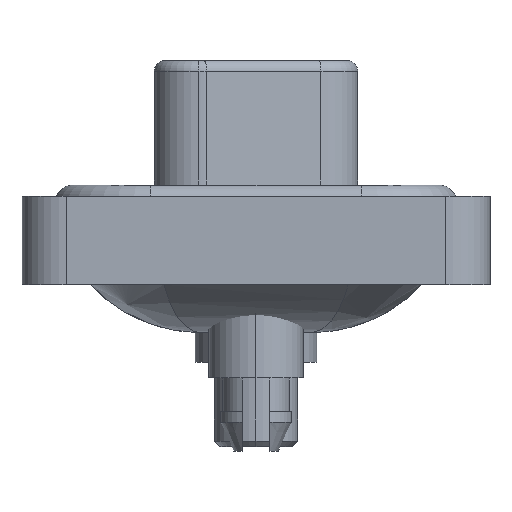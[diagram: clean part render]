
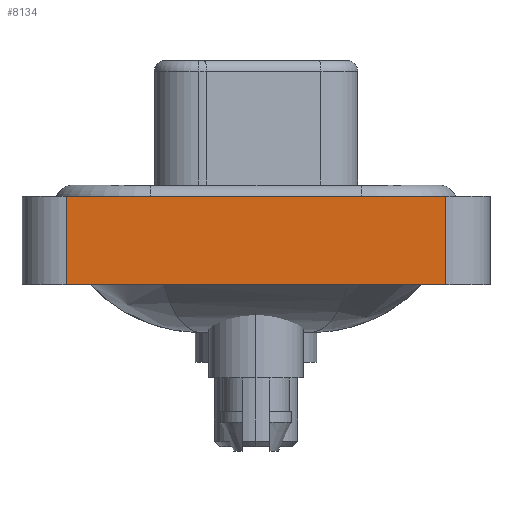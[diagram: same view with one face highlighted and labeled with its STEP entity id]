
A CAD part, left-side view. The second image highlights one B-rep face of the part: STEP entity #8134.
In plain terms, the highlighted planar face has unit normal (-1, 0, 0).
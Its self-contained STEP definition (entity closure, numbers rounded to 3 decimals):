
#729 = DIRECTION ( 'NONE',  ( 0., -1., 0. ) ) ;
#868 = DIRECTION ( 'NONE',  ( 0., 0., 1. ) ) ;
#1236 = AXIS2_PLACEMENT_3D ( 'NONE', #20802, #19509, #9401 ) ;
#2865 = CARTESIAN_POINT ( 'NONE',  ( -7.3, 8.55, 0.4 ) ) ;
#2893 = VERTEX_POINT ( 'NONE', #2865 ) ;
#3242 = ORIENTED_EDGE ( 'NONE', *, *, #5064, .F. ) ;
#3441 = VECTOR ( 'NONE', #729, 1000. ) ;
#3460 = VERTEX_POINT ( 'NONE', #5232 ) ;
#4652 = EDGE_CURVE ( 'NONE', #16499, #15998, #14033, .T. ) ;
#4703 = PLANE ( 'NONE',  #1236 ) ;
#5064 = EDGE_CURVE ( 'NONE', #3460, #2893, #7783, .T. ) ;
#5232 = CARTESIAN_POINT ( 'NONE',  ( -7.3, 8.55, -3.6 ) ) ;
#6170 = ORIENTED_EDGE ( 'NONE', *, *, #4652, .T. ) ;
#6194 = ORIENTED_EDGE ( 'NONE', *, *, #15832, .T. ) ;
#7319 = EDGE_CURVE ( 'NONE', #2893, #15998, #15734, .T. ) ;
#7783 = LINE ( 'NONE', #16155, #11412 ) ;
#8134 = ADVANCED_FACE ( 'NONE', ( #14066 ), #4703, .T. ) ;
#9253 = CARTESIAN_POINT ( 'NONE',  ( -7.3, -8.55, -3.6 ) ) ;
#9401 = DIRECTION ( 'NONE',  ( 0., 0., 1. ) ) ;
#10560 = CARTESIAN_POINT ( 'NONE',  ( -7.3, -8.55, -3.6 ) ) ;
#11108 = EDGE_LOOP ( 'NONE', ( #6170, #12699, #3242, #6194 ) ) ;
#11412 = VECTOR ( 'NONE', #19312, 1000. ) ;
#12194 = LINE ( 'NONE', #10560, #18953 ) ;
#12699 = ORIENTED_EDGE ( 'NONE', *, *, #7319, .F. ) ;
#13611 = DIRECTION ( 'NONE',  ( 0., -1., 0. ) ) ;
#14033 = LINE ( 'NONE', #9253, #20084 ) ;
#14066 = FACE_OUTER_BOUND ( 'NONE', #11108, .T. ) ;
#15734 = LINE ( 'NONE', #18997, #3441 ) ;
#15832 = EDGE_CURVE ( 'NONE', #3460, #16499, #12194, .T. ) ;
#15998 = VERTEX_POINT ( 'NONE', #20863 ) ;
#16155 = CARTESIAN_POINT ( 'NONE',  ( -7.3, 8.55, -3.6 ) ) ;
#16499 = VERTEX_POINT ( 'NONE', #18975 ) ;
#18953 = VECTOR ( 'NONE', #13611, 1000. ) ;
#18975 = CARTESIAN_POINT ( 'NONE',  ( -7.3, -8.55, -3.6 ) ) ;
#18997 = CARTESIAN_POINT ( 'NONE',  ( -7.3, -8.55, 0.4 ) ) ;
#19312 = DIRECTION ( 'NONE',  ( 0., 0., 1. ) ) ;
#19509 = DIRECTION ( 'NONE',  ( -1., 0., 0. ) ) ;
#20084 = VECTOR ( 'NONE', #868, 1000. ) ;
#20802 = CARTESIAN_POINT ( 'NONE',  ( -7.3, -8.55, -3.6 ) ) ;
#20863 = CARTESIAN_POINT ( 'NONE',  ( -7.3, -8.55, 0.4 ) ) ;
